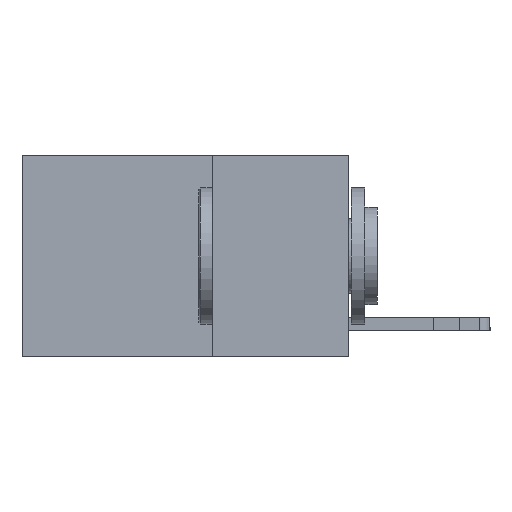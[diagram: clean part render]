
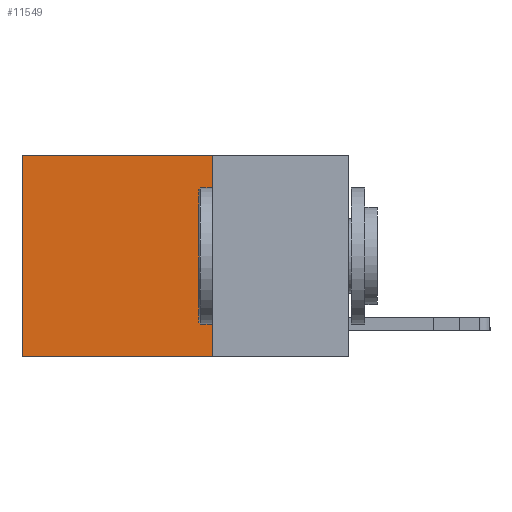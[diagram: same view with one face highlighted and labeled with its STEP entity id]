
A CAD part, left-side view. The second image highlights one B-rep face of the part: STEP entity #11549.
In plain terms, the highlighted planar face has unit normal (-1, 0, 0).
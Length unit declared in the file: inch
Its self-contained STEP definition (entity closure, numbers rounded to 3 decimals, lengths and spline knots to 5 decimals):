
#691 = CARTESIAN_POINT ( 'NONE',  ( 0.2625, 0.6, -0.37 ) ) ;
#989 = VECTOR ( 'NONE', #7991, 39.37008 ) ;
#1652 = VERTEX_POINT ( 'NONE', #6117 ) ;
#2130 = CARTESIAN_POINT ( 'NONE',  ( 0.2625, 0.25, 0. ) ) ;
#2425 = VECTOR ( 'NONE', #3066, 39.37008 ) ;
#2484 = EDGE_LOOP ( 'NONE', ( #12511, #8111, #13147, #11464 ) ) ;
#2500 = VERTEX_POINT ( 'NONE', #4254 ) ;
#2819 = FACE_OUTER_BOUND ( 'NONE', #2484, .T. ) ;
#2890 = PLANE ( 'NONE',  #4008 ) ;
#3063 = DIRECTION ( 'NONE',  ( 0., 1., 0. ) ) ;
#3066 = DIRECTION ( 'NONE',  ( 0., 1., 0. ) ) ;
#3995 = VECTOR ( 'NONE', #3063, 39.37008 ) ;
#4008 = AXIS2_PLACEMENT_3D ( 'NONE', #10445, #11698, #6081 ) ;
#4202 = EDGE_CURVE ( 'NONE', #2500, #8475, #4236, .T. ) ;
#4236 = LINE ( 'NONE', #9802, #2425 ) ;
#4254 = CARTESIAN_POINT ( 'NONE',  ( 0.2625, 0.25, -0.37 ) ) ;
#6081 = DIRECTION ( 'NONE',  ( 0., 0., -1. ) ) ;
#6117 = CARTESIAN_POINT ( 'NONE',  ( 0.2625, 0.6, 0. ) ) ;
#6590 = VECTOR ( 'NONE', #8644, 39.37008 ) ;
#6669 = CARTESIAN_POINT ( 'NONE',  ( 0.2625, 0.6, 0. ) ) ;
#7278 = LINE ( 'NONE', #9583, #3995 ) ;
#7991 = DIRECTION ( 'NONE',  ( 0., 0., -1. ) ) ;
#8111 = ORIENTED_EDGE ( 'NONE', *, *, #4202, .F. ) ;
#8475 = VERTEX_POINT ( 'NONE', #691 ) ;
#8644 = DIRECTION ( 'NONE',  ( 0., 0., -1. ) ) ;
#8704 = EDGE_CURVE ( 'NONE', #1652, #8475, #10205, .T. ) ;
#8926 = EDGE_CURVE ( 'NONE', #11004, #2500, #9752, .T. ) ;
#9583 = CARTESIAN_POINT ( 'NONE',  ( 0.2625, 0.25, 0. ) ) ;
#9752 = LINE ( 'NONE', #13230, #6590 ) ;
#9802 = CARTESIAN_POINT ( 'NONE',  ( 0.2625, 0.25, -0.37 ) ) ;
#10205 = LINE ( 'NONE', #6669, #989 ) ;
#10445 = CARTESIAN_POINT ( 'NONE',  ( 0.2625, 0.25, 0. ) ) ;
#11004 = VERTEX_POINT ( 'NONE', #2130 ) ;
#11339 = EDGE_CURVE ( 'NONE', #11004, #1652, #7278, .T. ) ;
#11464 = ORIENTED_EDGE ( 'NONE', *, *, #11339, .T. ) ;
#11549 = ADVANCED_FACE ( 'NONE', ( #2819 ), #2890, .F. ) ;
#11698 = DIRECTION ( 'NONE',  ( 1., 0., 0. ) ) ;
#12511 = ORIENTED_EDGE ( 'NONE', *, *, #8704, .T. ) ;
#13147 = ORIENTED_EDGE ( 'NONE', *, *, #8926, .F. ) ;
#13230 = CARTESIAN_POINT ( 'NONE',  ( 0.2625, 0.25, 0. ) ) ;
